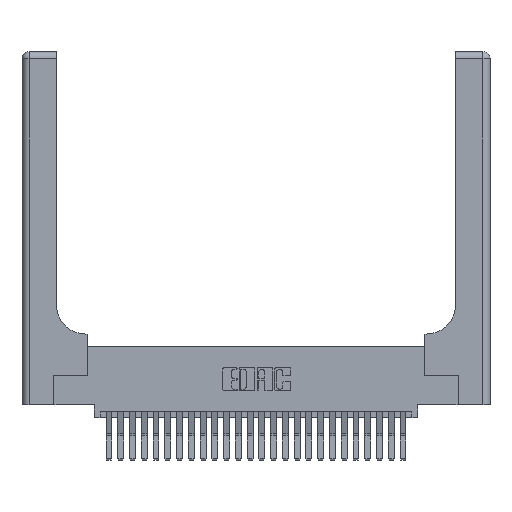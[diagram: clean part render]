
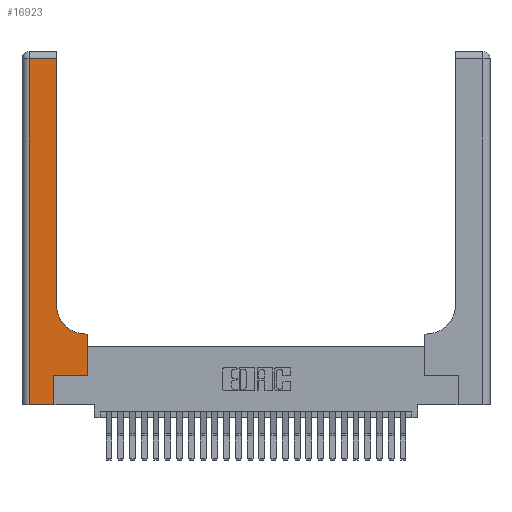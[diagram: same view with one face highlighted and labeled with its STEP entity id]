
A CAD part, top view. The second image highlights one B-rep face of the part: STEP entity #16923.
In plain terms, the highlighted planar face has unit normal (0, 0, 1).
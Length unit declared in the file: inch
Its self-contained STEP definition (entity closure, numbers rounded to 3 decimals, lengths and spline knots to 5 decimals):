
#56 = LINE ( 'NONE', #25330, #22387 ) ;
#758 = CARTESIAN_POINT ( 'NONE',  ( 0.269, 0., 0.37 ) ) ;
#1170 = LINE ( 'NONE', #21547, #25835 ) ;
#1275 = EDGE_CURVE ( 'NONE', #8568, #4829, #14346, .T. ) ;
#1459 = VECTOR ( 'NONE', #13035, 39.37008 ) ;
#1769 = VERTEX_POINT ( 'NONE', #11635 ) ;
#1941 = VERTEX_POINT ( 'NONE', #13680 ) ;
#2088 = DIRECTION ( 'NONE',  ( 1., 0., 0. ) ) ;
#2907 = VERTEX_POINT ( 'NONE', #3625 ) ;
#3625 = CARTESIAN_POINT ( 'NONE',  ( 0.5585, 0.6, 0.37 ) ) ;
#4829 = VERTEX_POINT ( 'NONE', #10995 ) ;
#5124 = DIRECTION ( 'NONE',  ( -1., 0., 0. ) ) ;
#5226 = LINE ( 'NONE', #14903, #11979 ) ;
#5305 = ORIENTED_EDGE ( 'NONE', *, *, #21105, .T. ) ;
#5761 = DIRECTION ( 'NONE',  ( 1., 0., 0. ) ) ;
#5789 = CARTESIAN_POINT ( 'NONE',  ( 0.5415, 0.6, 0.37 ) ) ;
#5852 = LINE ( 'NONE', #14241, #9878 ) ;
#6126 = CARTESIAN_POINT ( 'NONE',  ( 0.2915, 2.94, 0.37 ) ) ;
#7320 = DIRECTION ( 'NONE',  ( -1., 0., 0. ) ) ;
#7731 = DIRECTION ( 'NONE',  ( 0., 0., -1. ) ) ;
#8455 = EDGE_LOOP ( 'NONE', ( #20913, #5305, #25109, #12982, #25069, #15220, #11628, #23740, #24269 ) ) ;
#8541 = VECTOR ( 'NONE', #19197, 39.37008 ) ;
#8568 = VERTEX_POINT ( 'NONE', #17099 ) ;
#8594 = EDGE_CURVE ( 'NONE', #1941, #2907, #5226, .T. ) ;
#9070 = CARTESIAN_POINT ( 'NONE',  ( 0.269, 0., 0.37 ) ) ;
#9379 = CARTESIAN_POINT ( 'NONE',  ( 0., 3., 0.37 ) ) ;
#9481 = FACE_OUTER_BOUND ( 'NONE', #8455, .T. ) ;
#9656 = EDGE_CURVE ( 'NONE', #4829, #24508, #56, .T. ) ;
#9878 = VECTOR ( 'NONE', #16528, 39.37008 ) ;
#10547 = LINE ( 'NONE', #758, #21336 ) ;
#10995 = CARTESIAN_POINT ( 'NONE',  ( 0.06, 0., 0.37 ) ) ;
#11628 = ORIENTED_EDGE ( 'NONE', *, *, #8594, .T. ) ;
#11635 = CARTESIAN_POINT ( 'NONE',  ( 0.269, 0.25, 0.37 ) ) ;
#11979 = VECTOR ( 'NONE', #14993, 39.37008 ) ;
#12187 = CARTESIAN_POINT ( 'NONE',  ( 0.5415, 0.85, 0.37 ) ) ;
#12256 = CARTESIAN_POINT ( 'NONE',  ( 0.2915, 0.85, 0.37 ) ) ;
#12982 = ORIENTED_EDGE ( 'NONE', *, *, #9656, .T. ) ;
#13035 = DIRECTION ( 'NONE',  ( 0., 1., 0. ) ) ;
#13641 = DIRECTION ( 'NONE',  ( 0., 1., 0. ) ) ;
#13680 = CARTESIAN_POINT ( 'NONE',  ( 0.5585, 0.25, 0.37 ) ) ;
#13784 = EDGE_CURVE ( 'NONE', #19380, #23544, #19173, .T. ) ;
#13873 = CARTESIAN_POINT ( 'NONE',  ( 0., 2.94, 0.37 ) ) ;
#14241 = CARTESIAN_POINT ( 'NONE',  ( 0.2915, 0.6, 0.37 ) ) ;
#14346 = LINE ( 'NONE', #18813, #8541 ) ;
#14903 = CARTESIAN_POINT ( 'NONE',  ( 0.5585, 0.25, 0.37 ) ) ;
#14964 = EDGE_CURVE ( 'NONE', #23544, #27966, #18756, .T. ) ;
#14993 = DIRECTION ( 'NONE',  ( 0., 1., 0. ) ) ;
#15220 = ORIENTED_EDGE ( 'NONE', *, *, #26806, .T. ) ;
#16366 = EDGE_CURVE ( 'NONE', #24508, #1769, #10547, .T. ) ;
#16528 = DIRECTION ( 'NONE',  ( -1., 0., 0. ) ) ;
#16923 = ADVANCED_FACE ( 'NONE', ( #9481 ), #24634, .F. ) ;
#16939 = AXIS2_PLACEMENT_3D ( 'NONE', #9379, #22407, #5124 ) ;
#17099 = CARTESIAN_POINT ( 'NONE',  ( 0.06, 2.94, 0.37 ) ) ;
#17513 = CARTESIAN_POINT ( 'NONE',  ( 0.2915, 3., 0.37 ) ) ;
#18756 = LINE ( 'NONE', #17513, #1459 ) ;
#18813 = CARTESIAN_POINT ( 'NONE',  ( 0.06, 3., 0.37 ) ) ;
#19173 = CIRCLE ( 'NONE', #26955, 0.25 ) ;
#19197 = DIRECTION ( 'NONE',  ( 0., -1., 0. ) ) ;
#19380 = VERTEX_POINT ( 'NONE', #5789 ) ;
#20502 = DIRECTION ( 'NONE',  ( 1., 0., 0. ) ) ;
#20913 = ORIENTED_EDGE ( 'NONE', *, *, #14964, .T. ) ;
#21105 = EDGE_CURVE ( 'NONE', #27966, #8568, #22035, .T. ) ;
#21232 = EDGE_CURVE ( 'NONE', #2907, #19380, #5852, .T. ) ;
#21336 = VECTOR ( 'NONE', #13641, 39.37008 ) ;
#21547 = CARTESIAN_POINT ( 'NONE',  ( 0.269, 0.25, 0.37 ) ) ;
#22035 = LINE ( 'NONE', #13873, #25408 ) ;
#22387 = VECTOR ( 'NONE', #20502, 39.37008 ) ;
#22407 = DIRECTION ( 'NONE',  ( 0., 0., -1. ) ) ;
#23544 = VERTEX_POINT ( 'NONE', #12256 ) ;
#23740 = ORIENTED_EDGE ( 'NONE', *, *, #21232, .T. ) ;
#24269 = ORIENTED_EDGE ( 'NONE', *, *, #13784, .T. ) ;
#24508 = VERTEX_POINT ( 'NONE', #9070 ) ;
#24634 = PLANE ( 'NONE',  #16939 ) ;
#25069 = ORIENTED_EDGE ( 'NONE', *, *, #16366, .T. ) ;
#25109 = ORIENTED_EDGE ( 'NONE', *, *, #1275, .T. ) ;
#25330 = CARTESIAN_POINT ( 'NONE',  ( 0., 0., 0.37 ) ) ;
#25408 = VECTOR ( 'NONE', #7320, 39.37008 ) ;
#25835 = VECTOR ( 'NONE', #2088, 39.37008 ) ;
#26806 = EDGE_CURVE ( 'NONE', #1769, #1941, #1170, .T. ) ;
#26955 = AXIS2_PLACEMENT_3D ( 'NONE', #12187, #7731, #5761 ) ;
#27966 = VERTEX_POINT ( 'NONE', #6126 ) ;
